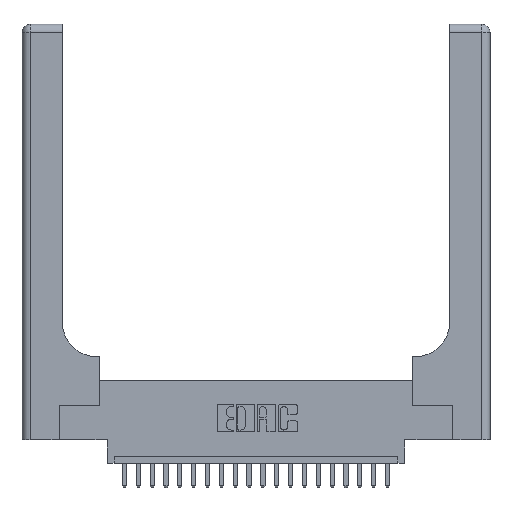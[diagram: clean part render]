
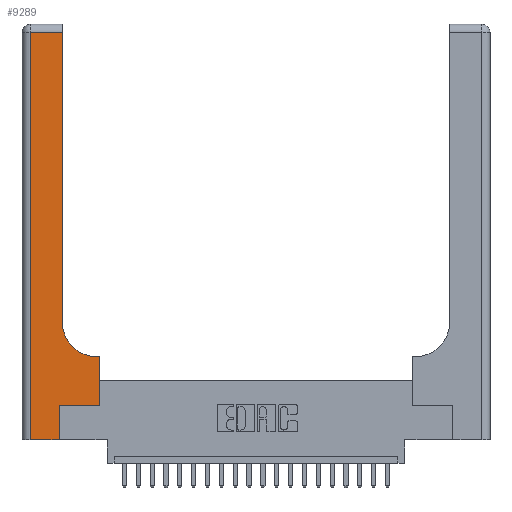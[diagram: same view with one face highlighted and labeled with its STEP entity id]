
A CAD part, top view. The second image highlights one B-rep face of the part: STEP entity #9289.
In plain terms, the highlighted planar face has unit normal (0, 0, 1).
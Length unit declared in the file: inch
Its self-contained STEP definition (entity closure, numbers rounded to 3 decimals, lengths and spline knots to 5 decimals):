
#180 = EDGE_LOOP ( 'NONE', ( #1786, #17239, #5294, #22563, #20595, #4422, #12457, #4807, #16241 ) ) ;
#189 = CARTESIAN_POINT ( 'NONE',  ( 0.5585, 0.25, 0.37 ) ) ;
#314 = DIRECTION ( 'NONE',  ( -1., 0., 0. ) ) ;
#788 = DIRECTION ( 'NONE',  ( 0., 1., 0. ) ) ;
#835 = LINE ( 'NONE', #23390, #11382 ) ;
#1374 = EDGE_CURVE ( 'NONE', #13644, #7179, #5991, .T. ) ;
#1636 = LINE ( 'NONE', #4691, #11912 ) ;
#1786 = ORIENTED_EDGE ( 'NONE', *, *, #22321, .T. ) ;
#1917 = CARTESIAN_POINT ( 'NONE',  ( 0.06, 2.94, 0.37 ) ) ;
#2617 = CARTESIAN_POINT ( 'NONE',  ( 0.269, 0.25, 0.37 ) ) ;
#3211 = VECTOR ( 'NONE', #788, 39.37008 ) ;
#4020 = VECTOR ( 'NONE', #314, 39.37008 ) ;
#4422 = ORIENTED_EDGE ( 'NONE', *, *, #1374, .T. ) ;
#4608 = VERTEX_POINT ( 'NONE', #7944 ) ;
#4691 = CARTESIAN_POINT ( 'NONE',  ( 0.269, 0., 0.37 ) ) ;
#4807 = ORIENTED_EDGE ( 'NONE', *, *, #5658, .T. ) ;
#4905 = VERTEX_POINT ( 'NONE', #19863 ) ;
#5294 = ORIENTED_EDGE ( 'NONE', *, *, #22875, .T. ) ;
#5453 = CARTESIAN_POINT ( 'NONE',  ( 0.5415, 0.85, 0.37 ) ) ;
#5658 = EDGE_CURVE ( 'NONE', #16020, #14744, #19426, .T. ) ;
#5991 = LINE ( 'NONE', #17040, #18175 ) ;
#6070 = CARTESIAN_POINT ( 'NONE',  ( 0.2915, 2.94, 0.37 ) ) ;
#6127 = CARTESIAN_POINT ( 'NONE',  ( 0.2915, 0.6, 0.37 ) ) ;
#6243 = DIRECTION ( 'NONE',  ( 1., 0., 0. ) ) ;
#6319 = VERTEX_POINT ( 'NONE', #6070 ) ;
#7179 = VERTEX_POINT ( 'NONE', #189 ) ;
#7494 = DIRECTION ( 'NONE',  ( 1., 0., 0. ) ) ;
#7526 = DIRECTION ( 'NONE',  ( 0., -1., 0. ) ) ;
#7535 = EDGE_CURVE ( 'NONE', #6319, #23440, #10020, .T. ) ;
#7830 = AXIS2_PLACEMENT_3D ( 'NONE', #10043, #18906, #11963 ) ;
#7944 = CARTESIAN_POINT ( 'NONE',  ( 0.2915, 0.85, 0.37 ) ) ;
#8214 = PLANE ( 'NONE',  #7830 ) ;
#8378 = DIRECTION ( 'NONE',  ( 0., 1., 0. ) ) ;
#9141 = DIRECTION ( 'NONE',  ( 0., 1., 0. ) ) ;
#9289 = ADVANCED_FACE ( 'NONE', ( #17557 ), #8214, .F. ) ;
#10020 = LINE ( 'NONE', #14750, #4020 ) ;
#10043 = CARTESIAN_POINT ( 'NONE',  ( 0., 3., 0.37 ) ) ;
#10320 = CARTESIAN_POINT ( 'NONE',  ( 0.5585, 0.6, 0.37 ) ) ;
#10828 = LINE ( 'NONE', #16542, #23245 ) ;
#11382 = VECTOR ( 'NONE', #7494, 39.37008 ) ;
#11421 = EDGE_CURVE ( 'NONE', #13277, #13644, #1636, .T. ) ;
#11514 = EDGE_CURVE ( 'NONE', #14744, #4608, #19533, .T. ) ;
#11670 = AXIS2_PLACEMENT_3D ( 'NONE', #5453, #11901, #6243 ) ;
#11901 = DIRECTION ( 'NONE',  ( 0., 0., -1. ) ) ;
#11912 = VECTOR ( 'NONE', #8378, 39.37008 ) ;
#11963 = DIRECTION ( 'NONE',  ( -1., 0., 0. ) ) ;
#12078 = DIRECTION ( 'NONE',  ( 1., 0., 0. ) ) ;
#12457 = ORIENTED_EDGE ( 'NONE', *, *, #18204, .T. ) ;
#13277 = VERTEX_POINT ( 'NONE', #17396 ) ;
#13644 = VERTEX_POINT ( 'NONE', #2617 ) ;
#14744 = VERTEX_POINT ( 'NONE', #16251 ) ;
#14750 = CARTESIAN_POINT ( 'NONE',  ( 0., 2.94, 0.37 ) ) ;
#15435 = LINE ( 'NONE', #22469, #3211 ) ;
#16020 = VERTEX_POINT ( 'NONE', #10320 ) ;
#16241 = ORIENTED_EDGE ( 'NONE', *, *, #11514, .T. ) ;
#16251 = CARTESIAN_POINT ( 'NONE',  ( 0.5415, 0.6, 0.37 ) ) ;
#16542 = CARTESIAN_POINT ( 'NONE',  ( 0.06, 3., 0.37 ) ) ;
#17040 = CARTESIAN_POINT ( 'NONE',  ( 0.269, 0.25, 0.37 ) ) ;
#17239 = ORIENTED_EDGE ( 'NONE', *, *, #7535, .T. ) ;
#17396 = CARTESIAN_POINT ( 'NONE',  ( 0.269, 0., 0.37 ) ) ;
#17557 = FACE_OUTER_BOUND ( 'NONE', #180, .T. ) ;
#17966 = CARTESIAN_POINT ( 'NONE',  ( 0.5585, 0.25, 0.37 ) ) ;
#18175 = VECTOR ( 'NONE', #12078, 39.37008 ) ;
#18204 = EDGE_CURVE ( 'NONE', #7179, #16020, #19301, .T. ) ;
#18906 = DIRECTION ( 'NONE',  ( 0., 0., -1. ) ) ;
#18998 = DIRECTION ( 'NONE',  ( -1., 0., 0. ) ) ;
#19301 = LINE ( 'NONE', #17966, #22963 ) ;
#19426 = LINE ( 'NONE', #6127, #21920 ) ;
#19533 = CIRCLE ( 'NONE', #11670, 0.25 ) ;
#19863 = CARTESIAN_POINT ( 'NONE',  ( 0.06, 0., 0.37 ) ) ;
#20595 = ORIENTED_EDGE ( 'NONE', *, *, #11421, .T. ) ;
#21920 = VECTOR ( 'NONE', #18998, 39.37008 ) ;
#22321 = EDGE_CURVE ( 'NONE', #4608, #6319, #15435, .T. ) ;
#22469 = CARTESIAN_POINT ( 'NONE',  ( 0.2915, 3., 0.37 ) ) ;
#22563 = ORIENTED_EDGE ( 'NONE', *, *, #23361, .T. ) ;
#22875 = EDGE_CURVE ( 'NONE', #23440, #4905, #10828, .T. ) ;
#22963 = VECTOR ( 'NONE', #9141, 39.37008 ) ;
#23245 = VECTOR ( 'NONE', #7526, 39.37008 ) ;
#23361 = EDGE_CURVE ( 'NONE', #4905, #13277, #835, .T. ) ;
#23390 = CARTESIAN_POINT ( 'NONE',  ( 0., 0., 0.37 ) ) ;
#23440 = VERTEX_POINT ( 'NONE', #1917 ) ;
